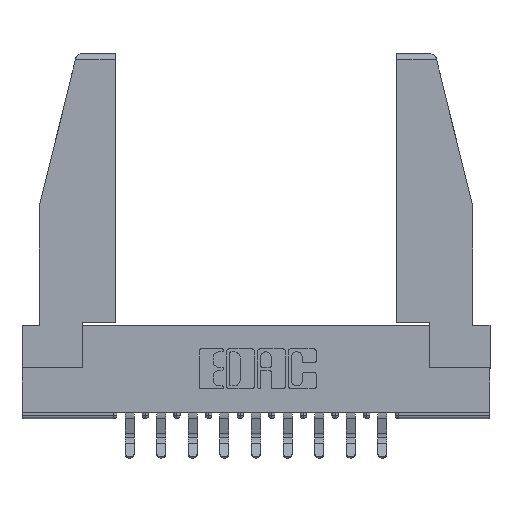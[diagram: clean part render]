
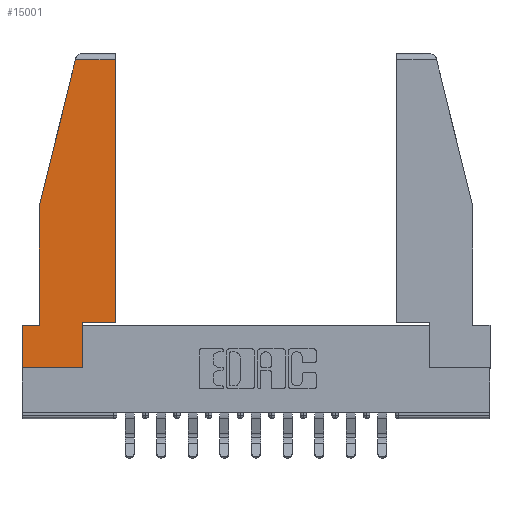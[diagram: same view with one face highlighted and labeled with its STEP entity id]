
A CAD part, top view. The second image highlights one B-rep face of the part: STEP entity #15001.
In plain terms, the highlighted planar face has unit normal (0, 0, 1).
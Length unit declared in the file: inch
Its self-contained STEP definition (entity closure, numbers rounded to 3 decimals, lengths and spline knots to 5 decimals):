
#491 = VERTEX_POINT ( 'NONE', #7094 ) ;
#500 = VERTEX_POINT ( 'NONE', #5863 ) ;
#535 = CARTESIAN_POINT ( 'NONE',  ( 0.297, 0.223, 0. ) ) ;
#618 = VECTOR ( 'NONE', #4139, 39.37008 ) ;
#1251 = VERTEX_POINT ( 'NONE', #1586 ) ;
#1539 = LINE ( 'NONE', #7439, #3474 ) ;
#1586 = CARTESIAN_POINT ( 'NONE',  ( 0., 0., 0. ) ) ;
#1896 = VERTEX_POINT ( 'NONE', #14214 ) ;
#2115 = ORIENTED_EDGE ( 'NONE', *, *, #4246, .T. ) ;
#2183 = DIRECTION ( 'NONE',  ( 1., 0., 0. ) ) ;
#2192 = VECTOR ( 'NONE', #11850, 39.37008 ) ;
#2953 = PLANE ( 'NONE',  #8323 ) ;
#3156 = LINE ( 'NONE', #7913, #618 ) ;
#3172 = ORIENTED_EDGE ( 'NONE', *, *, #12905, .T. ) ;
#3474 = VECTOR ( 'NONE', #15171, 39.37008 ) ;
#3677 = VERTEX_POINT ( 'NONE', #8498 ) ;
#3725 = ORIENTED_EDGE ( 'NONE', *, *, #4673, .T. ) ;
#3985 = ORIENTED_EDGE ( 'NONE', *, *, #15988, .T. ) ;
#4028 = CARTESIAN_POINT ( 'NONE',  ( 0.297, 0.223, 0. ) ) ;
#4139 = DIRECTION ( 'NONE',  ( -1., 0., 0. ) ) ;
#4246 = EDGE_CURVE ( 'NONE', #14422, #500, #9605, .T. ) ;
#4433 = VERTEX_POINT ( 'NONE', #12702 ) ;
#4673 = EDGE_CURVE ( 'NONE', #8788, #491, #8393, .T. ) ;
#4695 = DIRECTION ( 'NONE',  ( -1., 0., 0. ) ) ;
#4820 = VERTEX_POINT ( 'NONE', #14287 ) ;
#4841 = LINE ( 'NONE', #9460, #13221 ) ;
#5450 = DIRECTION ( 'NONE',  ( -0.239, -0.971, 0. ) ) ;
#5711 = DIRECTION ( 'NONE',  ( 0., -1., 0. ) ) ;
#5863 = CARTESIAN_POINT ( 'NONE',  ( 0.086, 0.8, 0. ) ) ;
#6210 = ORIENTED_EDGE ( 'NONE', *, *, #6674, .T. ) ;
#6674 = EDGE_CURVE ( 'NONE', #500, #1896, #4841, .T. ) ;
#6897 = ORIENTED_EDGE ( 'NONE', *, *, #11780, .T. ) ;
#6950 = LINE ( 'NONE', #11170, #11725 ) ;
#7094 = CARTESIAN_POINT ( 'NONE',  ( 0.461, 0.223, 0. ) ) ;
#7331 = EDGE_LOOP ( 'NONE', ( #13161, #11743, #2115, #6210, #3172, #6897, #3985, #14900, #3725 ) ) ;
#7439 = CARTESIAN_POINT ( 'NONE',  ( 0.461, 0.223, 0. ) ) ;
#7778 = FACE_OUTER_BOUND ( 'NONE', #7331, .T. ) ;
#7913 = CARTESIAN_POINT ( 'NONE',  ( 0., 0.21, 0. ) ) ;
#7946 = CARTESIAN_POINT ( 'NONE',  ( 0.271, 1.55, 0. ) ) ;
#7984 = VECTOR ( 'NONE', #4695, 39.37008 ) ;
#8323 = AXIS2_PLACEMENT_3D ( 'NONE', #14520, #15666, #15783 ) ;
#8393 = LINE ( 'NONE', #535, #8600 ) ;
#8431 = VECTOR ( 'NONE', #12522, 39.37008 ) ;
#8498 = CARTESIAN_POINT ( 'NONE',  ( 0.461, 1.52, 0. ) ) ;
#8600 = VECTOR ( 'NONE', #13232, 39.37008 ) ;
#8788 = VERTEX_POINT ( 'NONE', #4028 ) ;
#9126 = EDGE_CURVE ( 'NONE', #491, #3677, #1539, .T. ) ;
#9460 = CARTESIAN_POINT ( 'NONE',  ( 0.086, 0.8, 0. ) ) ;
#9605 = LINE ( 'NONE', #7946, #10997 ) ;
#9658 = EDGE_CURVE ( 'NONE', #4820, #8788, #12604, .T. ) ;
#10485 = CARTESIAN_POINT ( 'NONE',  ( 0., 0.21, 0. ) ) ;
#10764 = LINE ( 'NONE', #11063, #7984 ) ;
#10997 = VECTOR ( 'NONE', #5450, 39.37008 ) ;
#11063 = CARTESIAN_POINT ( 'NONE',  ( 0., 1.52, 0. ) ) ;
#11170 = CARTESIAN_POINT ( 'NONE',  ( 0., 0., 0. ) ) ;
#11725 = VECTOR ( 'NONE', #2183, 39.37008 ) ;
#11743 = ORIENTED_EDGE ( 'NONE', *, *, #14659, .T. ) ;
#11780 = EDGE_CURVE ( 'NONE', #4433, #1251, #13347, .T. ) ;
#11850 = DIRECTION ( 'NONE',  ( 0., -1., 0. ) ) ;
#12085 = CARTESIAN_POINT ( 'NONE',  ( 0.2636, 1.52, 0. ) ) ;
#12474 = CARTESIAN_POINT ( 'NONE',  ( 0.297, 0., 0. ) ) ;
#12522 = DIRECTION ( 'NONE',  ( 0., 1., 0. ) ) ;
#12604 = LINE ( 'NONE', #12474, #8431 ) ;
#12702 = CARTESIAN_POINT ( 'NONE',  ( 0., 0.21, 0. ) ) ;
#12905 = EDGE_CURVE ( 'NONE', #1896, #4433, #3156, .T. ) ;
#13161 = ORIENTED_EDGE ( 'NONE', *, *, #9126, .T. ) ;
#13221 = VECTOR ( 'NONE', #5711, 39.37008 ) ;
#13232 = DIRECTION ( 'NONE',  ( 1., 0., 0. ) ) ;
#13347 = LINE ( 'NONE', #10485, #2192 ) ;
#14214 = CARTESIAN_POINT ( 'NONE',  ( 0.086, 0.21, 0. ) ) ;
#14287 = CARTESIAN_POINT ( 'NONE',  ( 0.297, 0., 0. ) ) ;
#14422 = VERTEX_POINT ( 'NONE', #12085 ) ;
#14520 = CARTESIAN_POINT ( 'NONE',  ( 0., 0., 0. ) ) ;
#14659 = EDGE_CURVE ( 'NONE', #3677, #14422, #10764, .T. ) ;
#14900 = ORIENTED_EDGE ( 'NONE', *, *, #9658, .T. ) ;
#15001 = ADVANCED_FACE ( 'NONE', ( #7778 ), #2953, .T. ) ;
#15171 = DIRECTION ( 'NONE',  ( 0., 1., 0. ) ) ;
#15666 = DIRECTION ( 'NONE',  ( 0., 0., 1. ) ) ;
#15783 = DIRECTION ( 'NONE',  ( 1., 0., 0. ) ) ;
#15988 = EDGE_CURVE ( 'NONE', #1251, #4820, #6950, .T. ) ;
